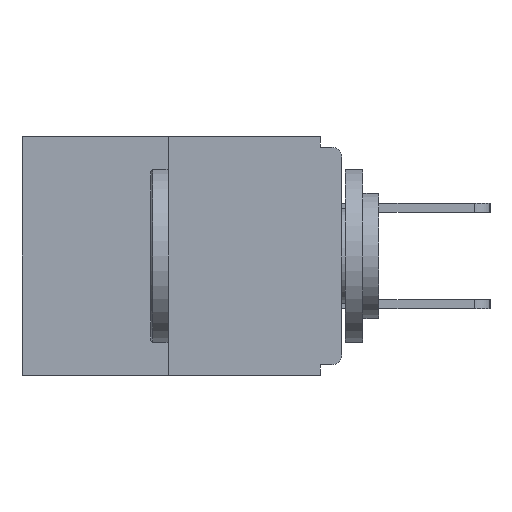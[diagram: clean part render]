
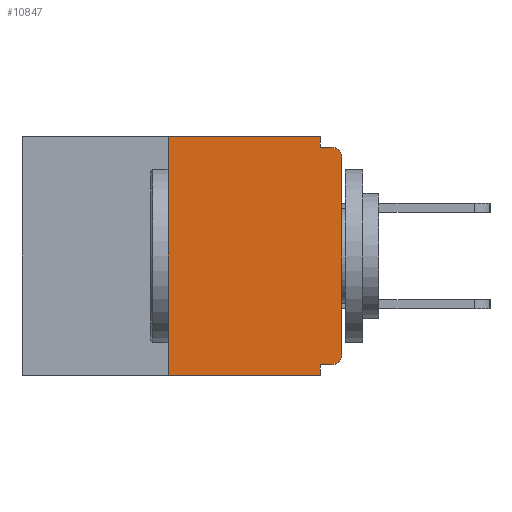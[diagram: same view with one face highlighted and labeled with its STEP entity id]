
A CAD part, left-side view. The second image highlights one B-rep face of the part: STEP entity #10847.
In plain terms, the highlighted planar face has unit normal (-1, 0, 0).
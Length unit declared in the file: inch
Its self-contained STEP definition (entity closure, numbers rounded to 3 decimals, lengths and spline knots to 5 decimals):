
#205 = EDGE_CURVE ( 'NONE', #10216, #6238, #6621, .T. ) ;
#293 = DIRECTION ( 'NONE',  ( 0., 1., 0. ) ) ;
#1006 = ORIENTED_EDGE ( 'NONE', *, *, #12304, .T. ) ;
#1143 = CARTESIAN_POINT ( 'NONE',  ( 0., 0.015, -0.328 ) ) ;
#1860 = CARTESIAN_POINT ( 'NONE',  ( 0., 0.031, 0. ) ) ;
#2107 = CARTESIAN_POINT ( 'NONE',  ( 0., 0.25, 0. ) ) ;
#2122 = LINE ( 'NONE', #5726, #9945 ) ;
#2210 = CARTESIAN_POINT ( 'NONE',  ( 0., 0.46, -0.343 ) ) ;
#2245 = CARTESIAN_POINT ( 'NONE',  ( 0., 0.031, -0.343 ) ) ;
#2298 = EDGE_CURVE ( 'NONE', #10216, #3154, #5476, .T. ) ;
#2629 = CARTESIAN_POINT ( 'NONE',  ( 0., 0.031, -0.343 ) ) ;
#2883 = ORIENTED_EDGE ( 'NONE', *, *, #11847, .F. ) ;
#2920 = ORIENTED_EDGE ( 'NONE', *, *, #7094, .F. ) ;
#3154 = VERTEX_POINT ( 'NONE', #10084 ) ;
#3588 = EDGE_CURVE ( 'NONE', #7921, #8848, #10789, .T. ) ;
#3644 = PLANE ( 'NONE',  #9060 ) ;
#3775 = ORIENTED_EDGE ( 'NONE', *, *, #205, .F. ) ;
#3828 = DIRECTION ( 'NONE',  ( 0., 0., -1. ) ) ;
#4030 = DIRECTION ( 'NONE',  ( 0., 0., -1. ) ) ;
#4528 = VECTOR ( 'NONE', #10759, 39.37008 ) ;
#4716 = EDGE_CURVE ( 'NONE', #6366, #9474, #10269, .T. ) ;
#4723 = DIRECTION ( 'NONE',  ( 0., 0., -1. ) ) ;
#4889 = CARTESIAN_POINT ( 'NONE',  ( 0., 0.031, 0. ) ) ;
#5174 = ORIENTED_EDGE ( 'NONE', *, *, #5176, .T. ) ;
#5176 = EDGE_CURVE ( 'NONE', #3154, #7921, #2122, .T. ) ;
#5355 = LINE ( 'NONE', #2629, #13050 ) ;
#5404 = FACE_OUTER_BOUND ( 'NONE', #11984, .T. ) ;
#5426 = DIRECTION ( 'NONE',  ( 0., 0., 1. ) ) ;
#5439 = VECTOR ( 'NONE', #293, 39.37008 ) ;
#5476 = CIRCLE ( 'NONE', #9907, 0.015 ) ;
#5532 = LINE ( 'NONE', #2210, #4528 ) ;
#5583 = ORIENTED_EDGE ( 'NONE', *, *, #12388, .F. ) ;
#5726 = CARTESIAN_POINT ( 'NONE',  ( 0., 0., 0. ) ) ;
#6086 = VECTOR ( 'NONE', #3828, 39.37008 ) ;
#6168 = ORIENTED_EDGE ( 'NONE', *, *, #9896, .F. ) ;
#6238 = VERTEX_POINT ( 'NONE', #8243 ) ;
#6366 = VERTEX_POINT ( 'NONE', #4889 ) ;
#6621 = LINE ( 'NONE', #12999, #5439 ) ;
#6632 = VECTOR ( 'NONE', #7235, 39.37008 ) ;
#6712 = LINE ( 'NONE', #11196, #10210 ) ;
#6939 = AXIS2_PLACEMENT_3D ( 'NONE', #12320, #7267, #4030 ) ;
#7094 = EDGE_CURVE ( 'NONE', #9401, #6366, #6712, .T. ) ;
#7235 = DIRECTION ( 'NONE',  ( 0., -1., 0. ) ) ;
#7267 = DIRECTION ( 'NONE',  ( -1., 0., 0. ) ) ;
#7813 = CARTESIAN_POINT ( 'NONE',  ( 0., 0.46, 0. ) ) ;
#7921 = VERTEX_POINT ( 'NONE', #10717 ) ;
#8155 = DIRECTION ( 'NONE',  ( -1., 0., 0. ) ) ;
#8243 = CARTESIAN_POINT ( 'NONE',  ( 0., 0.031, -0.328 ) ) ;
#8519 = CARTESIAN_POINT ( 'NONE',  ( 0., 0.031, -0.015 ) ) ;
#8552 = VERTEX_POINT ( 'NONE', #2245 ) ;
#8848 = VERTEX_POINT ( 'NONE', #13204 ) ;
#8925 = VECTOR ( 'NONE', #5426, 39.37008 ) ;
#8972 = DIRECTION ( 'NONE',  ( 1., 0., 0. ) ) ;
#8979 = LINE ( 'NONE', #10437, #6632 ) ;
#9029 = DIRECTION ( 'NONE',  ( 0., 0., 1. ) ) ;
#9060 = AXIS2_PLACEMENT_3D ( 'NONE', #7813, #8972, #4723 ) ;
#9342 = ORIENTED_EDGE ( 'NONE', *, *, #4716, .F. ) ;
#9401 = VERTEX_POINT ( 'NONE', #2107 ) ;
#9474 = VERTEX_POINT ( 'NONE', #8519 ) ;
#9896 = EDGE_CURVE ( 'NONE', #9474, #8848, #8979, .T. ) ;
#9907 = AXIS2_PLACEMENT_3D ( 'NONE', #11403, #8155, #12479 ) ;
#9945 = VECTOR ( 'NONE', #9029, 39.37008 ) ;
#10084 = CARTESIAN_POINT ( 'NONE',  ( 0., 0., -0.313 ) ) ;
#10090 = DIRECTION ( 'NONE',  ( 0., 0., -1. ) ) ;
#10131 = VERTEX_POINT ( 'NONE', #10887 ) ;
#10210 = VECTOR ( 'NONE', #13550, 39.37008 ) ;
#10216 = VERTEX_POINT ( 'NONE', #1143 ) ;
#10269 = LINE ( 'NONE', #1860, #6086 ) ;
#10437 = CARTESIAN_POINT ( 'NONE',  ( 0., 0., -0.015 ) ) ;
#10708 = CARTESIAN_POINT ( 'NONE',  ( 0., 0.25, 0. ) ) ;
#10717 = CARTESIAN_POINT ( 'NONE',  ( 0., 0., -0.03 ) ) ;
#10759 = DIRECTION ( 'NONE',  ( 0., -1., 0. ) ) ;
#10789 = CIRCLE ( 'NONE', #6939, 0.015 ) ;
#10847 = ADVANCED_FACE ( 'NONE', ( #5404 ), #3644, .F. ) ;
#10887 = CARTESIAN_POINT ( 'NONE',  ( 0., 0.25, -0.343 ) ) ;
#11196 = CARTESIAN_POINT ( 'NONE',  ( 0., 0.46, 0. ) ) ;
#11403 = CARTESIAN_POINT ( 'NONE',  ( 0., 0.015, -0.313 ) ) ;
#11557 = LINE ( 'NONE', #10708, #8925 ) ;
#11847 = EDGE_CURVE ( 'NONE', #10131, #9401, #11557, .T. ) ;
#11984 = EDGE_LOOP ( 'NONE', ( #2920, #2883, #1006, #5583, #3775, #13068, #5174, #13436, #6168, #9342 ) ) ;
#12304 = EDGE_CURVE ( 'NONE', #10131, #8552, #5532, .T. ) ;
#12320 = CARTESIAN_POINT ( 'NONE',  ( 0., 0.015, -0.03 ) ) ;
#12388 = EDGE_CURVE ( 'NONE', #6238, #8552, #5355, .T. ) ;
#12479 = DIRECTION ( 'NONE',  ( 0., 0., -1. ) ) ;
#12999 = CARTESIAN_POINT ( 'NONE',  ( 0., 0., -0.328 ) ) ;
#13050 = VECTOR ( 'NONE', #10090, 39.37008 ) ;
#13068 = ORIENTED_EDGE ( 'NONE', *, *, #2298, .T. ) ;
#13204 = CARTESIAN_POINT ( 'NONE',  ( 0., 0.015, -0.015 ) ) ;
#13436 = ORIENTED_EDGE ( 'NONE', *, *, #3588, .T. ) ;
#13550 = DIRECTION ( 'NONE',  ( 0., -1., 0. ) ) ;
